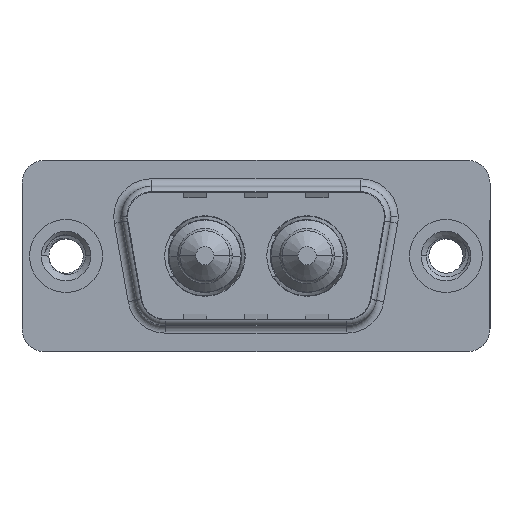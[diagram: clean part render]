
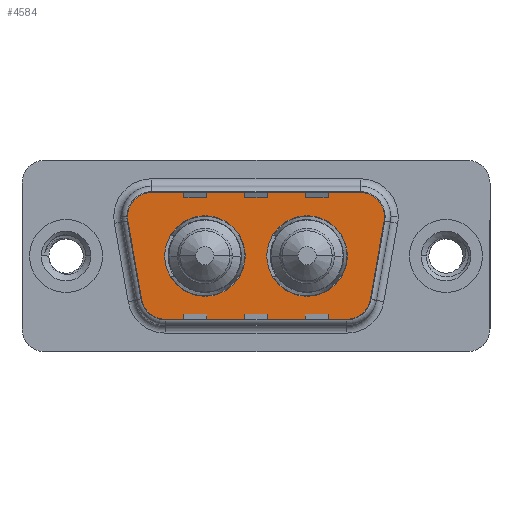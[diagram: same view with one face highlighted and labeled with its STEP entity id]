
A CAD part, top view. The second image highlights one B-rep face of the part: STEP entity #4584.
In plain terms, the highlighted planar face has unit normal (0, 0, 1).
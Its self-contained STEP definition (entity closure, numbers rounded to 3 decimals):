
#9 = DIRECTION ( 'NONE',  ( 0., 0., 1. ) ) ;
#39 = EDGE_CURVE ( 'NONE', #2894, #2438, #11175, .T. ) ;
#109 = CARTESIAN_POINT ( 'NONE',  ( 19.564, 2.9, 0. ) ) ;
#185 = DIRECTION ( 'NONE',  ( 0., 0., 1. ) ) ;
#230 = AXIS2_PLACEMENT_3D ( 'NONE', #7936, #185, #12607 ) ;
#294 = CARTESIAN_POINT ( 'NONE',  ( 3.466, 2.553, 0. ) ) ;
#318 = AXIS2_PLACEMENT_3D ( 'NONE', #11976, #6896, #1473 ) ;
#323 = CARTESIAN_POINT ( 'NONE',  ( 6.459, -2.9, 0. ) ) ;
#348 = DIRECTION ( 'NONE',  ( 0., 0., 1. ) ) ;
#571 = CARTESIAN_POINT ( 'NONE',  ( 15.86, 0., 0. ) ) ;
#720 = VERTEX_POINT ( 'NONE', #5860 ) ;
#791 = ORIENTED_EDGE ( 'NONE', *, *, #3019, .F. ) ;
#1073 = CARTESIAN_POINT ( 'NONE',  ( 18.541, -2.9, 0. ) ) ;
#1080 = CARTESIAN_POINT ( 'NONE',  ( 4.489, -3.247, 0. ) ) ;
#1184 = VERTEX_POINT ( 'NONE', #7905 ) ;
#1190 = CIRCLE ( 'NONE', #5208, 2.65 ) ;
#1473 = DIRECTION ( 'NONE',  ( 1., 0., 0. ) ) ;
#1539 = CARTESIAN_POINT ( 'NONE',  ( 13.21, 0., 0. ) ) ;
#1697 = ORIENTED_EDGE ( 'NONE', *, *, #6736, .T. ) ;
#1761 = AXIS2_PLACEMENT_3D ( 'NONE', #10370, #6934, #6579 ) ;
#1867 = VECTOR ( 'NONE', #2364, 1000. ) ;
#1963 = AXIS2_PLACEMENT_3D ( 'NONE', #12081, #5583, #13155 ) ;
#2010 = DIRECTION ( 'NONE',  ( 0., 0., 1. ) ) ;
#2223 = LINE ( 'NONE', #11154, #1867 ) ;
#2364 = DIRECTION ( 'NONE',  ( 0.174, 0.985, 0. ) ) ;
#2417 = CIRCLE ( 'NONE', #4594, 2. ) ;
#2438 = VERTEX_POINT ( 'NONE', #8595 ) ;
#2539 = LINE ( 'NONE', #10135, #10602 ) ;
#2894 = VERTEX_POINT ( 'NONE', #9965 ) ;
#2923 = CIRCLE ( 'NONE', #12006, 2. ) ;
#2945 = AXIS2_PLACEMENT_3D ( 'NONE', #6676, #9, #7778 ) ;
#2963 = CARTESIAN_POINT ( 'NONE',  ( 21.534, 2.553, 0. ) ) ;
#3019 = EDGE_CURVE ( 'NONE', #6309, #7163, #6792, .T. ) ;
#3524 = ORIENTED_EDGE ( 'NONE', *, *, #7353, .T. ) ;
#3684 = CARTESIAN_POINT ( 'NONE',  ( 5.436, 4.9, 0. ) ) ;
#3705 = VERTEX_POINT ( 'NONE', #1539 ) ;
#3725 = EDGE_CURVE ( 'NONE', #9597, #8832, #5463, .T. ) ;
#3780 = VERTEX_POINT ( 'NONE', #4263 ) ;
#3879 = CARTESIAN_POINT ( 'NONE',  ( 15.86, 0., 0. ) ) ;
#3908 = EDGE_CURVE ( 'NONE', #720, #3780, #5951, .T. ) ;
#4125 = EDGE_CURVE ( 'NONE', #11549, #3705, #4219, .T. ) ;
#4219 = CIRCLE ( 'NONE', #8384, 2.65 ) ;
#4263 = CARTESIAN_POINT ( 'NONE',  ( 20.511, -3.247, 0. ) ) ;
#4285 = VERTEX_POINT ( 'NONE', #6244 ) ;
#4380 = CARTESIAN_POINT ( 'NONE',  ( 3.466, 2.553, 0. ) ) ;
#4462 = ORIENTED_EDGE ( 'NONE', *, *, #8091, .T. ) ;
#4584 = ADVANCED_FACE ( 'NONE', ( #6608, #9126, #6290 ), #9101, .T. ) ;
#4594 = AXIS2_PLACEMENT_3D ( 'NONE', #109, #348, #7913 ) ;
#4615 = DIRECTION ( 'NONE',  ( 0., 0., 1. ) ) ;
#4951 = AXIS2_PLACEMENT_3D ( 'NONE', #1073, #5633, #6377 ) ;
#4997 = DIRECTION ( 'NONE',  ( 1., 0., 0. ) ) ;
#5005 = DIRECTION ( 'NONE',  ( 1., 0., 0. ) ) ;
#5208 = AXIS2_PLACEMENT_3D ( 'NONE', #3879, #11500, #5005 ) ;
#5463 = LINE ( 'NONE', #294, #11214 ) ;
#5563 = CIRCLE ( 'NONE', #1963, 2.65 ) ;
#5583 = DIRECTION ( 'NONE',  ( 0., 0., 1. ) ) ;
#5609 = EDGE_CURVE ( 'NONE', #1184, #2894, #2417, .T. ) ;
#5633 = DIRECTION ( 'NONE',  ( 0., 0., 1. ) ) ;
#5649 = ORIENTED_EDGE ( 'NONE', *, *, #9877, .F. ) ;
#5753 = DIRECTION ( 'NONE',  ( 1., 0., 0. ) ) ;
#5860 = CARTESIAN_POINT ( 'NONE',  ( 18.541, -4.9, 0. ) ) ;
#5916 = ORIENTED_EDGE ( 'NONE', *, *, #39, .T. ) ;
#5951 = CIRCLE ( 'NONE', #230, 2. ) ;
#5973 = DIRECTION ( 'NONE',  ( 0.174, -0.985, 0. ) ) ;
#6084 = CIRCLE ( 'NONE', #1761, 2. ) ;
#6244 = CARTESIAN_POINT ( 'NONE',  ( 6.459, -4.9, 0. ) ) ;
#6270 = EDGE_CURVE ( 'NONE', #2438, #9597, #6084, .T. ) ;
#6290 = FACE_OUTER_BOUND ( 'NONE', #8465, .T. ) ;
#6309 = VERTEX_POINT ( 'NONE', #13764 ) ;
#6377 = DIRECTION ( 'NONE',  ( 1., 0., 0. ) ) ;
#6554 = ORIENTED_EDGE ( 'NONE', *, *, #3908, .T. ) ;
#6579 = DIRECTION ( 'NONE',  ( 1., 0., 0. ) ) ;
#6608 = FACE_BOUND ( 'NONE', #11445, .T. ) ;
#6676 = CARTESIAN_POINT ( 'NONE',  ( 19.564, 2.9, 0. ) ) ;
#6736 = EDGE_CURVE ( 'NONE', #3780, #10518, #2223, .T. ) ;
#6792 = CIRCLE ( 'NONE', #318, 2.65 ) ;
#6896 = DIRECTION ( 'NONE',  ( 0., 0., 1. ) ) ;
#6934 = DIRECTION ( 'NONE',  ( 0., 0., 1. ) ) ;
#7112 = DIRECTION ( 'NONE',  ( -1., 0., 0. ) ) ;
#7163 = VERTEX_POINT ( 'NONE', #10647 ) ;
#7245 = EDGE_LOOP ( 'NONE', ( #791, #10221 ) ) ;
#7297 = DIRECTION ( 'NONE',  ( -1., 0., 0. ) ) ;
#7353 = EDGE_CURVE ( 'NONE', #8832, #4285, #2923, .T. ) ;
#7778 = DIRECTION ( 'NONE',  ( -1., 0., 0. ) ) ;
#7905 = CARTESIAN_POINT ( 'NONE',  ( 21.564, 2.9, 0. ) ) ;
#7913 = DIRECTION ( 'NONE',  ( -1., 0., 0. ) ) ;
#7936 = CARTESIAN_POINT ( 'NONE',  ( 18.541, -2.9, 0. ) ) ;
#8091 = EDGE_CURVE ( 'NONE', #4285, #720, #2539, .T. ) ;
#8384 = AXIS2_PLACEMENT_3D ( 'NONE', #571, #4615, #4997 ) ;
#8465 = EDGE_LOOP ( 'NONE', ( #6554, #1697, #11262, #10586, #5916, #13687, #8842, #3524, #4462 ) ) ;
#8595 = CARTESIAN_POINT ( 'NONE',  ( 5.436, 4.9, 0. ) ) ;
#8832 = VERTEX_POINT ( 'NONE', #1080 ) ;
#8842 = ORIENTED_EDGE ( 'NONE', *, *, #3725, .T. ) ;
#9101 = PLANE ( 'NONE',  #4951 ) ;
#9126 = FACE_BOUND ( 'NONE', #7245, .T. ) ;
#9151 = EDGE_CURVE ( 'NONE', #7163, #6309, #5563, .T. ) ;
#9597 = VERTEX_POINT ( 'NONE', #4380 ) ;
#9877 = EDGE_CURVE ( 'NONE', #3705, #11549, #1190, .T. ) ;
#9965 = CARTESIAN_POINT ( 'NONE',  ( 19.564, 4.9, 0. ) ) ;
#10135 = CARTESIAN_POINT ( 'NONE',  ( 6.459, -4.9, 0. ) ) ;
#10221 = ORIENTED_EDGE ( 'NONE', *, *, #9151, .F. ) ;
#10370 = CARTESIAN_POINT ( 'NONE',  ( 5.436, 2.9, 0. ) ) ;
#10518 = VERTEX_POINT ( 'NONE', #2963 ) ;
#10586 = ORIENTED_EDGE ( 'NONE', *, *, #5609, .T. ) ;
#10602 = VECTOR ( 'NONE', #5753, 1000. ) ;
#10647 = CARTESIAN_POINT ( 'NONE',  ( 6.49, 0., 0. ) ) ;
#10824 = VECTOR ( 'NONE', #7297, 1000. ) ;
#11110 = CIRCLE ( 'NONE', #2945, 2. ) ;
#11154 = CARTESIAN_POINT ( 'NONE',  ( 21.534, 2.553, 0. ) ) ;
#11175 = LINE ( 'NONE', #3684, #10824 ) ;
#11214 = VECTOR ( 'NONE', #5973, 1000. ) ;
#11262 = ORIENTED_EDGE ( 'NONE', *, *, #11659, .T. ) ;
#11445 = EDGE_LOOP ( 'NONE', ( #11533, #5649 ) ) ;
#11500 = DIRECTION ( 'NONE',  ( 0., 0., 1. ) ) ;
#11533 = ORIENTED_EDGE ( 'NONE', *, *, #4125, .F. ) ;
#11549 = VERTEX_POINT ( 'NONE', #11937 ) ;
#11659 = EDGE_CURVE ( 'NONE', #10518, #1184, #11110, .T. ) ;
#11937 = CARTESIAN_POINT ( 'NONE',  ( 18.51, 0., 0. ) ) ;
#11976 = CARTESIAN_POINT ( 'NONE',  ( 9.14, 0., 0. ) ) ;
#12006 = AXIS2_PLACEMENT_3D ( 'NONE', #323, #2010, #7112 ) ;
#12081 = CARTESIAN_POINT ( 'NONE',  ( 9.14, 0., 0. ) ) ;
#12607 = DIRECTION ( 'NONE',  ( 1., 0., 0. ) ) ;
#13155 = DIRECTION ( 'NONE',  ( 1., 0., 0. ) ) ;
#13687 = ORIENTED_EDGE ( 'NONE', *, *, #6270, .T. ) ;
#13764 = CARTESIAN_POINT ( 'NONE',  ( 11.79, 0., 0. ) ) ;
